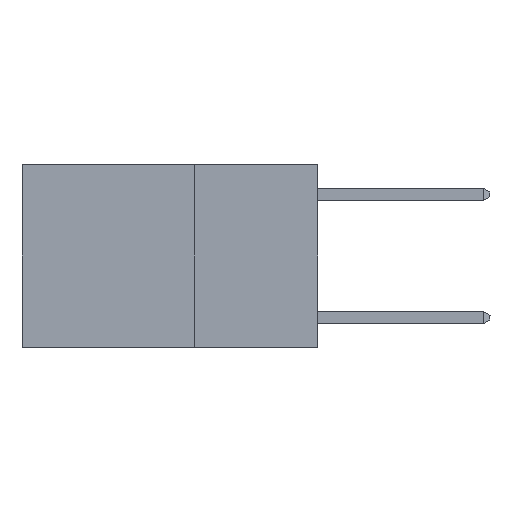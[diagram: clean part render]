
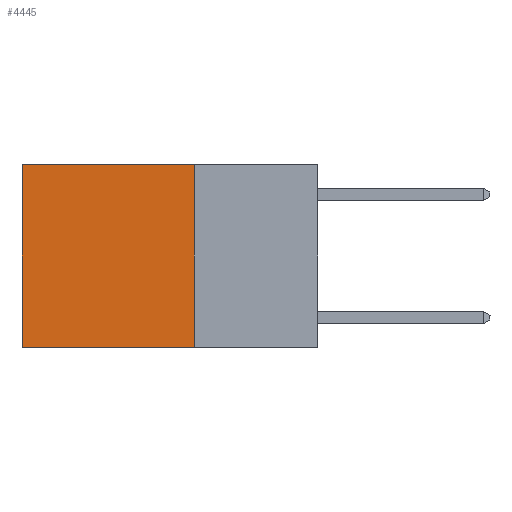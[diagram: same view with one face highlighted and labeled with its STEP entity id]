
A CAD part, left-side view. The second image highlights one B-rep face of the part: STEP entity #4445.
In plain terms, the highlighted planar face has unit normal (-1, 0, 0).
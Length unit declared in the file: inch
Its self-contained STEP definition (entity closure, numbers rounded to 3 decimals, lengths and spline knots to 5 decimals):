
#165 = VERTEX_POINT ( 'NONE', #2860 ) ;
#226 = LINE ( 'NONE', #3718, #4681 ) ;
#419 = DIRECTION ( 'NONE',  ( 0., 1., 0. ) ) ;
#554 = ORIENTED_EDGE ( 'NONE', *, *, #8019, .T. ) ;
#569 = DIRECTION ( 'NONE',  ( 0., 0., -1. ) ) ;
#1200 = CARTESIAN_POINT ( 'NONE',  ( 0.2625, 0.25, -0.37 ) ) ;
#1227 = EDGE_CURVE ( 'NONE', #165, #5028, #2789, .T. ) ;
#1462 = CARTESIAN_POINT ( 'NONE',  ( 0.2625, 0.25, -0.37 ) ) ;
#1646 = EDGE_CURVE ( 'NONE', #5028, #4189, #3714, .T. ) ;
#1983 = PLANE ( 'NONE',  #7283 ) ;
#2215 = ORIENTED_EDGE ( 'NONE', *, *, #2455, .T. ) ;
#2455 = EDGE_CURVE ( 'NONE', #165, #5355, #226, .T. ) ;
#2789 = LINE ( 'NONE', #6712, #6594 ) ;
#2860 = CARTESIAN_POINT ( 'NONE',  ( 0.2625, 0.25, 0. ) ) ;
#3276 = VECTOR ( 'NONE', #569, 39.37008 ) ;
#3328 = DIRECTION ( 'NONE',  ( 0., 0., -1. ) ) ;
#3714 = LINE ( 'NONE', #1200, #8736 ) ;
#3718 = CARTESIAN_POINT ( 'NONE',  ( 0.2625, 0.25, 0. ) ) ;
#4093 = DIRECTION ( 'NONE',  ( 1., 0., 0. ) ) ;
#4189 = VERTEX_POINT ( 'NONE', #6151 ) ;
#4308 = CARTESIAN_POINT ( 'NONE',  ( 0.2625, 0.6, 0. ) ) ;
#4445 = ADVANCED_FACE ( 'NONE', ( #4536 ), #1983, .F. ) ;
#4536 = FACE_OUTER_BOUND ( 'NONE', #7562, .T. ) ;
#4605 = CARTESIAN_POINT ( 'NONE',  ( 0.2625, 0.25, 0. ) ) ;
#4681 = VECTOR ( 'NONE', #5105, 39.37008 ) ;
#4804 = DIRECTION ( 'NONE',  ( 0., 0., -1. ) ) ;
#5028 = VERTEX_POINT ( 'NONE', #1462 ) ;
#5105 = DIRECTION ( 'NONE',  ( 0., 1., 0. ) ) ;
#5355 = VERTEX_POINT ( 'NONE', #4308 ) ;
#6151 = CARTESIAN_POINT ( 'NONE',  ( 0.2625, 0.6, -0.37 ) ) ;
#6594 = VECTOR ( 'NONE', #3328, 39.37008 ) ;
#6712 = CARTESIAN_POINT ( 'NONE',  ( 0.2625, 0.25, 0. ) ) ;
#6888 = LINE ( 'NONE', #8656, #3276 ) ;
#7283 = AXIS2_PLACEMENT_3D ( 'NONE', #4605, #4093, #4804 ) ;
#7562 = EDGE_LOOP ( 'NONE', ( #554, #7665, #8508, #2215 ) ) ;
#7665 = ORIENTED_EDGE ( 'NONE', *, *, #1646, .F. ) ;
#8019 = EDGE_CURVE ( 'NONE', #5355, #4189, #6888, .T. ) ;
#8508 = ORIENTED_EDGE ( 'NONE', *, *, #1227, .F. ) ;
#8656 = CARTESIAN_POINT ( 'NONE',  ( 0.2625, 0.6, 0. ) ) ;
#8736 = VECTOR ( 'NONE', #419, 39.37008 ) ;
